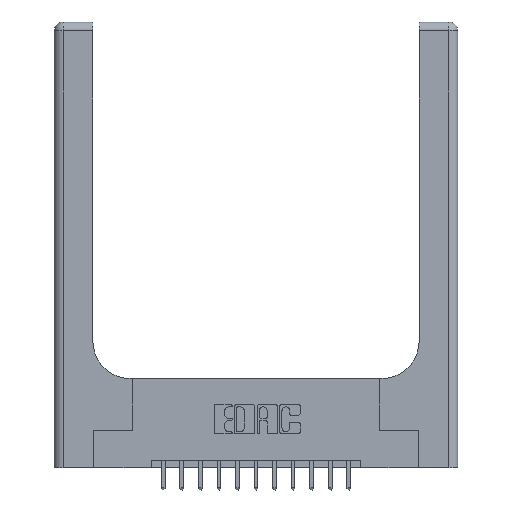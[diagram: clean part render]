
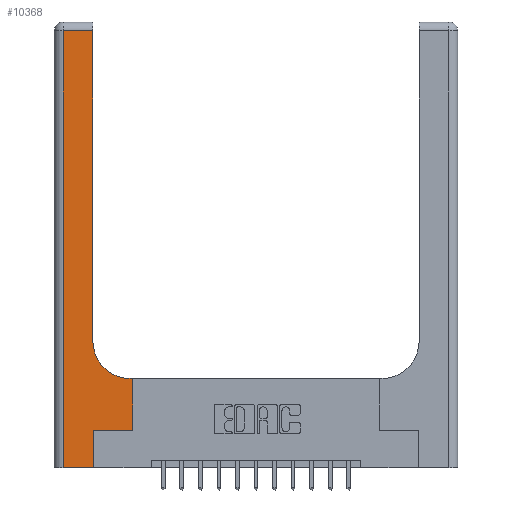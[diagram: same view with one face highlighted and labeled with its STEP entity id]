
A CAD part, top view. The second image highlights one B-rep face of the part: STEP entity #10368.
In plain terms, the highlighted planar face has unit normal (0, 0, 1).
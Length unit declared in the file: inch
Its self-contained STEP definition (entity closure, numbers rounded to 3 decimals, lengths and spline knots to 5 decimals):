
#32 = CARTESIAN_POINT ( 'NONE',  ( 0.528, 0.25, 0.37 ) ) ;
#663 = LINE ( 'NONE', #5909, #15954 ) ;
#1173 = ORIENTED_EDGE ( 'NONE', *, *, #4700, .T. ) ;
#1267 = VERTEX_POINT ( 'NONE', #9098 ) ;
#1319 = CARTESIAN_POINT ( 'NONE',  ( 0.26, 2.94, 0.37 ) ) ;
#1595 = ORIENTED_EDGE ( 'NONE', *, *, #9231, .T. ) ;
#1806 = VERTEX_POINT ( 'NONE', #4078 ) ;
#2168 = VERTEX_POINT ( 'NONE', #7939 ) ;
#2499 = CIRCLE ( 'NONE', #7439, 0.25 ) ;
#2553 = VERTEX_POINT ( 'NONE', #11673 ) ;
#2618 = LINE ( 'NONE', #32, #4677 ) ;
#2985 = DIRECTION ( 'NONE',  ( 1., 0., 0. ) ) ;
#3098 = CARTESIAN_POINT ( 'NONE',  ( 0.06, 3., 0.37 ) ) ;
#3133 = DIRECTION ( 'NONE',  ( 0., 1., 0. ) ) ;
#3304 = VECTOR ( 'NONE', #13578, 39.37008 ) ;
#4004 = VERTEX_POINT ( 'NONE', #10397 ) ;
#4073 = EDGE_CURVE ( 'NONE', #2168, #4004, #8093, .T. ) ;
#4078 = CARTESIAN_POINT ( 'NONE',  ( 0.26, 0.85, 0.37 ) ) ;
#4127 = EDGE_CURVE ( 'NONE', #2553, #13016, #5599, .T. ) ;
#4244 = CARTESIAN_POINT ( 'NONE',  ( 0.26, 3., 0.37 ) ) ;
#4677 = VECTOR ( 'NONE', #13017, 39.37008 ) ;
#4700 = EDGE_CURVE ( 'NONE', #4004, #1806, #2499, .T. ) ;
#4988 = VECTOR ( 'NONE', #9221, 39.37008 ) ;
#5291 = LINE ( 'NONE', #16806, #12673 ) ;
#5363 = ORIENTED_EDGE ( 'NONE', *, *, #4127, .T. ) ;
#5506 = DIRECTION ( 'NONE',  ( 0., 0., -1. ) ) ;
#5599 = LINE ( 'NONE', #3098, #3304 ) ;
#5677 = CARTESIAN_POINT ( 'NONE',  ( 0.26, 0.6, 0.37 ) ) ;
#5751 = CARTESIAN_POINT ( 'NONE',  ( 0.51, 0.85, 0.37 ) ) ;
#5909 = CARTESIAN_POINT ( 'NONE',  ( 0.265, 0.25, 0.37 ) ) ;
#5912 = CARTESIAN_POINT ( 'NONE',  ( 0., 3., 0.37 ) ) ;
#5930 = ORIENTED_EDGE ( 'NONE', *, *, #4073, .T. ) ;
#6174 = CARTESIAN_POINT ( 'NONE',  ( 0.06, 0., 0.37 ) ) ;
#6491 = VERTEX_POINT ( 'NONE', #8830 ) ;
#6880 = DIRECTION ( 'NONE',  ( 0., 0., -1. ) ) ;
#7312 = EDGE_CURVE ( 'NONE', #13016, #12419, #15665, .T. ) ;
#7439 = AXIS2_PLACEMENT_3D ( 'NONE', #5751, #6880, #13652 ) ;
#7865 = DIRECTION ( 'NONE',  ( 0., 1., 0. ) ) ;
#7939 = CARTESIAN_POINT ( 'NONE',  ( 0.528, 0.6, 0.37 ) ) ;
#8036 = CARTESIAN_POINT ( 'NONE',  ( 0.265, 0., 0.37 ) ) ;
#8093 = LINE ( 'NONE', #5677, #9083 ) ;
#8177 = PLANE ( 'NONE',  #15129 ) ;
#8258 = DIRECTION ( 'NONE',  ( -1., 0., 0. ) ) ;
#8830 = CARTESIAN_POINT ( 'NONE',  ( 0.528, 0.25, 0.37 ) ) ;
#8898 = EDGE_LOOP ( 'NONE', ( #15402, #15837, #5363, #10765, #10038, #1595, #13571, #5930, #1173 ) ) ;
#9083 = VECTOR ( 'NONE', #8258, 39.37008 ) ;
#9098 = CARTESIAN_POINT ( 'NONE',  ( 0.265, 0.25, 0.37 ) ) ;
#9221 = DIRECTION ( 'NONE',  ( 1., 0., 0. ) ) ;
#9231 = EDGE_CURVE ( 'NONE', #1267, #6491, #663, .T. ) ;
#9410 = VECTOR ( 'NONE', #3133, 39.37008 ) ;
#9741 = LINE ( 'NONE', #4244, #9410 ) ;
#9926 = EDGE_CURVE ( 'NONE', #6491, #2168, #2618, .T. ) ;
#9991 = DIRECTION ( 'NONE',  ( -1., 0., 0. ) ) ;
#10038 = ORIENTED_EDGE ( 'NONE', *, *, #12331, .T. ) ;
#10368 = ADVANCED_FACE ( 'NONE', ( #13331 ), #8177, .F. ) ;
#10397 = CARTESIAN_POINT ( 'NONE',  ( 0.51, 0.6, 0.37 ) ) ;
#10765 = ORIENTED_EDGE ( 'NONE', *, *, #7312, .T. ) ;
#11535 = LINE ( 'NONE', #16621, #15772 ) ;
#11673 = CARTESIAN_POINT ( 'NONE',  ( 0.06, 2.94, 0.37 ) ) ;
#11957 = DIRECTION ( 'NONE',  ( -1., 0., 0. ) ) ;
#12331 = EDGE_CURVE ( 'NONE', #12419, #1267, #5291, .T. ) ;
#12419 = VERTEX_POINT ( 'NONE', #8036 ) ;
#12673 = VECTOR ( 'NONE', #7865, 39.37008 ) ;
#13016 = VERTEX_POINT ( 'NONE', #6174 ) ;
#13017 = DIRECTION ( 'NONE',  ( 0., 1., 0. ) ) ;
#13331 = FACE_OUTER_BOUND ( 'NONE', #8898, .T. ) ;
#13571 = ORIENTED_EDGE ( 'NONE', *, *, #9926, .T. ) ;
#13578 = DIRECTION ( 'NONE',  ( 0., -1., 0. ) ) ;
#13584 = EDGE_CURVE ( 'NONE', #1806, #14947, #9741, .T. ) ;
#13652 = DIRECTION ( 'NONE',  ( 1., 0., 0. ) ) ;
#14754 = EDGE_CURVE ( 'NONE', #14947, #2553, #11535, .T. ) ;
#14947 = VERTEX_POINT ( 'NONE', #1319 ) ;
#15129 = AXIS2_PLACEMENT_3D ( 'NONE', #5912, #5506, #11957 ) ;
#15402 = ORIENTED_EDGE ( 'NONE', *, *, #13584, .T. ) ;
#15503 = CARTESIAN_POINT ( 'NONE',  ( 0., 0., 0.37 ) ) ;
#15665 = LINE ( 'NONE', #15503, #4988 ) ;
#15772 = VECTOR ( 'NONE', #9991, 39.37008 ) ;
#15837 = ORIENTED_EDGE ( 'NONE', *, *, #14754, .T. ) ;
#15954 = VECTOR ( 'NONE', #2985, 39.37008 ) ;
#16621 = CARTESIAN_POINT ( 'NONE',  ( 0., 2.94, 0.37 ) ) ;
#16806 = CARTESIAN_POINT ( 'NONE',  ( 0.265, 0., 0.37 ) ) ;
